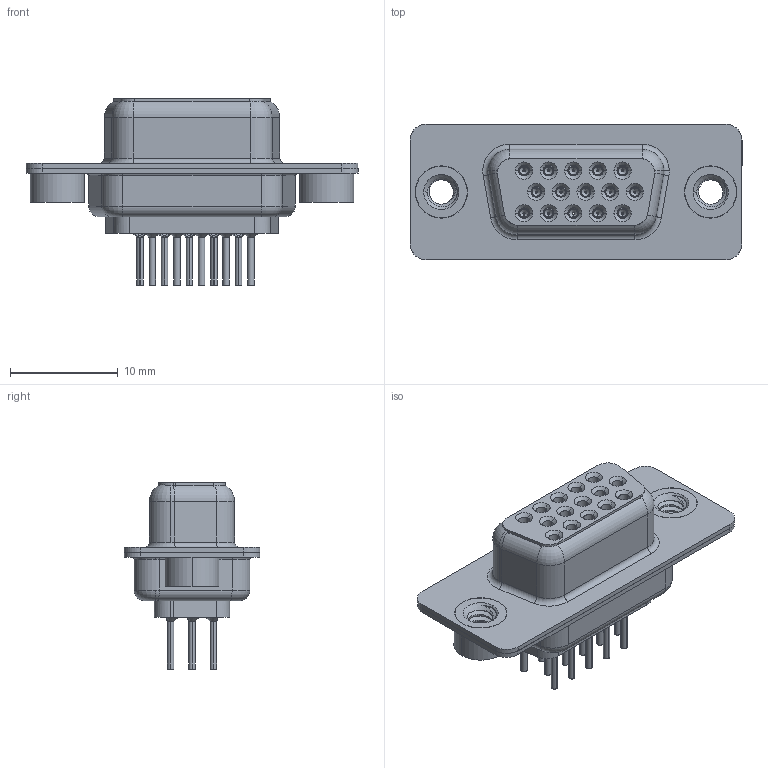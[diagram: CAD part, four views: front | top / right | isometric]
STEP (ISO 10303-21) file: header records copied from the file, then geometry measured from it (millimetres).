
FILE_DESCRIPTION (( 'STEP AP203' ), '1' );
FILE_NAME ('638-015-230-042.STEP', '2019-05-14T12:09:10', ( '' ), ( '' ), 'SwSTEP 2.0', 'SolidWorks 2016', '' );
FILE_SCHEMA (( 'CONFIG_CONTROL_DESIGN' ));
Length unit declared in the file: millimetre
Products named in the file (8): 638 Housing_15 Contacts; 638 Shell Front_15 Contacts; 638 Shell Rear_15 Contacts; 638 Contact Row 1_30L; 638 Contact Row 2_30L; 638 Contact Row 3_30L; 638 4-40 Threaded Rivet; 638-015-230-042
Assembly tree (20 placements, depth 2):
  638-015-230-042
    638 Housing_15 Contacts
    638 Shell Front_15 Contacts
    638 Shell Rear_15 Contacts
    638 Contact Row 1_30L  x5
    638 Contact Row 2_30L  x5
    638 Contact Row 3_30L  x5
    638 4-40 Threaded Rivet  x2
Bounding box: 30.81 x 12.6 x 17.3 mm (x, y, z)
Volume: 1576.7 mm3; surface area: 5598.3 mm2
Topology: 20 solids, 20 shells, 2184 faces, 5545 edges, 3442 vertices
Faces by surface type: cylinder 632, plane 532, torus 447, bspline 306, cone 267
Entity records: 28410 total; most frequent: CARTESIAN_POINT 9098, DIRECTION 3864, ORIENTED_EDGE 3794, EDGE_CURVE 1897, AXIS2_PLACEMENT_3D 1604, VERTEX_POINT 1188, EDGE_LOOP 875, CIRCLE 867
